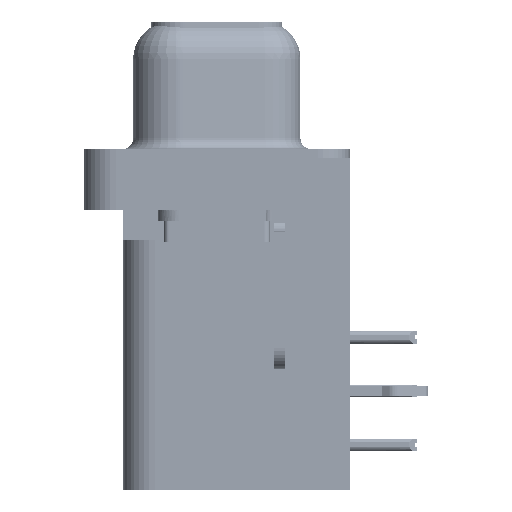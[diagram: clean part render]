
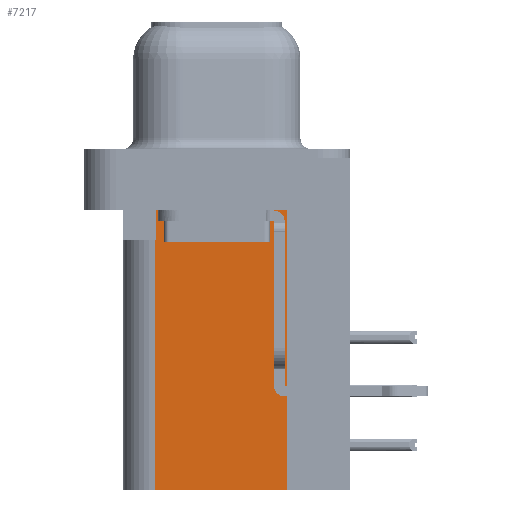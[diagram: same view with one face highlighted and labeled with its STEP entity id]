
A CAD part, left-side view. The second image highlights one B-rep face of the part: STEP entity #7217.
In plain terms, the highlighted planar face has unit normal (-1, 0, 0).
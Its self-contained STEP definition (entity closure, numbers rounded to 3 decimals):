
#82 = DIRECTION ( 'NONE',  ( 0., 0., 1. ) ) ;
#508 = EDGE_LOOP ( 'NONE', ( #4592, #15204, #33146, #39585, #2831, #6655 ) ) ;
#582 = EDGE_CURVE ( 'NONE', #12249, #1851, #23445, .T. ) ;
#909 = CARTESIAN_POINT ( 'NONE',  ( 3.7, -3.295, -15.7 ) ) ;
#971 = DIRECTION ( 'NONE',  ( 0., 0., 1. ) ) ;
#1851 = VERTEX_POINT ( 'NONE', #32713 ) ;
#2425 = DIRECTION ( 'NONE',  ( 0., 0., -1. ) ) ;
#2831 = ORIENTED_EDGE ( 'NONE', *, *, #24285, .F. ) ;
#3748 = VECTOR ( 'NONE', #971, 1000. ) ;
#4046 = CARTESIAN_POINT ( 'NONE',  ( 3.7, 2.925, -15.7 ) ) ;
#4421 = VERTEX_POINT ( 'NONE', #33214 ) ;
#4592 = ORIENTED_EDGE ( 'NONE', *, *, #33186, .T. ) ;
#6546 = VECTOR ( 'NONE', #32307, 1000. ) ;
#6655 = ORIENTED_EDGE ( 'NONE', *, *, #582, .T. ) ;
#7217 = ADVANCED_FACE ( 'NONE', ( #17057 ), #35829, .F. ) ;
#7695 = LINE ( 'NONE', #33972, #25283 ) ;
#7976 = EDGE_CURVE ( 'NONE', #4421, #17096, #7695, .T. ) ;
#8931 = DIRECTION ( 'NONE',  ( 0., 1., 0. ) ) ;
#11362 = EDGE_CURVE ( 'NONE', #14748, #38461, #40836, .T. ) ;
#11633 = DIRECTION ( 'NONE',  ( 0., 0., -1. ) ) ;
#12064 = CARTESIAN_POINT ( 'NONE',  ( 3.7, -3.295, -15.7 ) ) ;
#12249 = VERTEX_POINT ( 'NONE', #12064 ) ;
#14089 = LINE ( 'NONE', #26471, #32625 ) ;
#14093 = VECTOR ( 'NONE', #82, 1000. ) ;
#14748 = VERTEX_POINT ( 'NONE', #4046 ) ;
#14938 = CARTESIAN_POINT ( 'NONE',  ( 3.7, -3.295, -2.5 ) ) ;
#15204 = ORIENTED_EDGE ( 'NONE', *, *, #7976, .T. ) ;
#17057 = FACE_OUTER_BOUND ( 'NONE', #508, .T. ) ;
#17096 = VERTEX_POINT ( 'NONE', #44065 ) ;
#18551 = CARTESIAN_POINT ( 'NONE',  ( 3.7, -3.295, -15.7 ) ) ;
#20499 = CARTESIAN_POINT ( 'NONE',  ( 3.7, 2.925, -3.9 ) ) ;
#23445 = LINE ( 'NONE', #909, #14093 ) ;
#24285 = EDGE_CURVE ( 'NONE', #12249, #14748, #35056, .T. ) ;
#24966 = CARTESIAN_POINT ( 'NONE',  ( 3.7, -3.295, -15.7 ) ) ;
#25283 = VECTOR ( 'NONE', #2425, 1000. ) ;
#25641 = CARTESIAN_POINT ( 'NONE',  ( 3.7, 2.925, -15.7 ) ) ;
#26471 = CARTESIAN_POINT ( 'NONE',  ( 3.7, 0., -3.9 ) ) ;
#28496 = DIRECTION ( 'NONE',  ( 0., 1., 0. ) ) ;
#29691 = EDGE_CURVE ( 'NONE', #17096, #38461, #14089, .T. ) ;
#32307 = DIRECTION ( 'NONE',  ( 0., 1., 0. ) ) ;
#32540 = DIRECTION ( 'NONE',  ( 1., 0., 0. ) ) ;
#32625 = VECTOR ( 'NONE', #8931, 1000. ) ;
#32713 = CARTESIAN_POINT ( 'NONE',  ( 3.7, -3.295, -2.5 ) ) ;
#33146 = ORIENTED_EDGE ( 'NONE', *, *, #29691, .T. ) ;
#33186 = EDGE_CURVE ( 'NONE', #1851, #4421, #43505, .T. ) ;
#33202 = AXIS2_PLACEMENT_3D ( 'NONE', #18551, #32540, #11633 ) ;
#33214 = CARTESIAN_POINT ( 'NONE',  ( 3.7, 2.895, -2.5 ) ) ;
#33972 = CARTESIAN_POINT ( 'NONE',  ( 3.7, 2.895, -3.9 ) ) ;
#35056 = LINE ( 'NONE', #24966, #39357 ) ;
#35829 = PLANE ( 'NONE',  #33202 ) ;
#38461 = VERTEX_POINT ( 'NONE', #20499 ) ;
#39357 = VECTOR ( 'NONE', #28496, 1000. ) ;
#39585 = ORIENTED_EDGE ( 'NONE', *, *, #11362, .F. ) ;
#40836 = LINE ( 'NONE', #25641, #3748 ) ;
#43505 = LINE ( 'NONE', #14938, #6546 ) ;
#44065 = CARTESIAN_POINT ( 'NONE',  ( 3.7, 2.895, -3.9 ) ) ;
